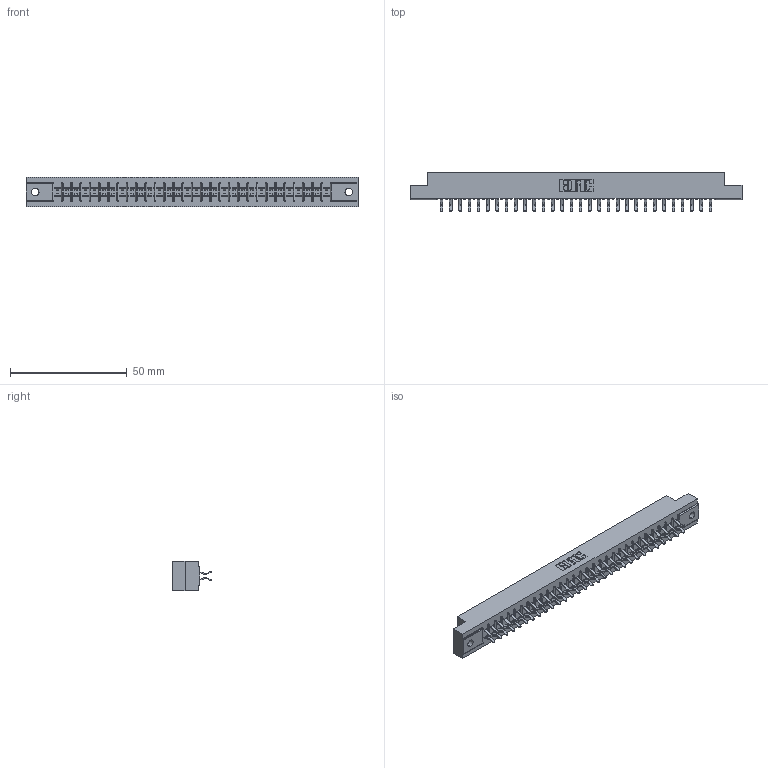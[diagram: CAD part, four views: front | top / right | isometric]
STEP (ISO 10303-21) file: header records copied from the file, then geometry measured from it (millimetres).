
FILE_DESCRIPTION (( 'STEP AP203' ), '1' );
FILE_NAME ('315-060-556-202.STEP', '2019-09-10T20:05:28', ( '' ), ( '' ), 'SwSTEP 2.0', 'SolidWorks 2016', '' );
FILE_SCHEMA (( 'CONFIG_CONTROL_DESIGN' ));
Length unit declared in the file: inch
Products named in the file (3): 305 Part_.128 Dia; 315-060-556-202; 305-290-001_556
Assembly tree (61 placements, depth 2):
  315-060-556-202
    305 Part_.128 Dia
    305-290-001_556  x60
Bounding box: 141.88 x 16.64 x 12.7 mm (x, y, z)
Volume: 14687.9 mm3; surface area: 18150.6 mm2
Topology: 61 solids, 61 shells, 3476 faces, 10006 edges, 6508 vertices
Faces by surface type: plane 1928, cylinder 1428, sphere 120
Entity records: 34167 total; most frequent: CARTESIAN_POINT 5656, ORIENTED_EDGE 5612, DIRECTION 5484, EDGE_CURVE 2806, LINE 2252, VECTOR 2252, VERTEX_POINT 1788, AXIS2_PLACEMENT_3D 1616
